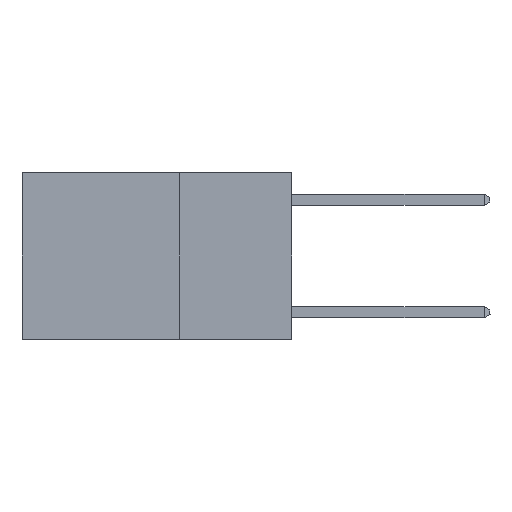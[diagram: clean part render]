
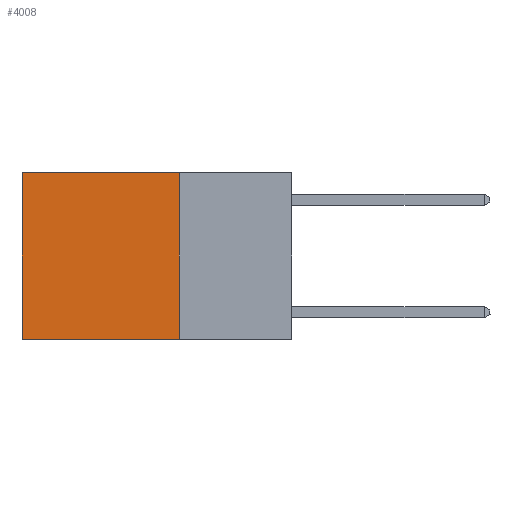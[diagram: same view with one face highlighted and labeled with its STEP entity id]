
A CAD part, left-side view. The second image highlights one B-rep face of the part: STEP entity #4008.
In plain terms, the highlighted planar face has unit normal (-1, 0, 0).
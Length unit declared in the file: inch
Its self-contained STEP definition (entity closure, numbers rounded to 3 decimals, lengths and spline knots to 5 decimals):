
#190 = VECTOR ( 'NONE', #16484, 39.37008 ) ;
#302 = CARTESIAN_POINT ( 'NONE',  ( 0.2625, 0.6, 0. ) ) ;
#377 = CARTESIAN_POINT ( 'NONE',  ( 0.2625, 0.6, -0.37 ) ) ;
#729 = EDGE_CURVE ( 'NONE', #3782, #8922, #2511, .T. ) ;
#951 = DIRECTION ( 'NONE',  ( 0., 0., -1. ) ) ;
#1135 = VECTOR ( 'NONE', #10407, 39.37008 ) ;
#2511 = LINE ( 'NONE', #17663, #1135 ) ;
#3301 = EDGE_CURVE ( 'NONE', #3782, #17445, #7290, .T. ) ;
#3782 = VERTEX_POINT ( 'NONE', #13985 ) ;
#4008 = ADVANCED_FACE ( 'NONE', ( #11550 ), #12716, .F. ) ;
#4341 = DIRECTION ( 'NONE',  ( 0., 1., 0. ) ) ;
#5199 = VERTEX_POINT ( 'NONE', #377 ) ;
#5431 = AXIS2_PLACEMENT_3D ( 'NONE', #18724, #9845, #951 ) ;
#5867 = CARTESIAN_POINT ( 'NONE',  ( 0.2625, 0.25, 0. ) ) ;
#6741 = ORIENTED_EDGE ( 'NONE', *, *, #8431, .F. ) ;
#6955 = ORIENTED_EDGE ( 'NONE', *, *, #729, .F. ) ;
#7290 = LINE ( 'NONE', #5867, #190 ) ;
#8431 = EDGE_CURVE ( 'NONE', #8922, #5199, #19445, .T. ) ;
#8922 = VERTEX_POINT ( 'NONE', #10956 ) ;
#9041 = ORIENTED_EDGE ( 'NONE', *, *, #3301, .T. ) ;
#9845 = DIRECTION ( 'NONE',  ( 1., 0., 0. ) ) ;
#10407 = DIRECTION ( 'NONE',  ( 0., 0., -1. ) ) ;
#10956 = CARTESIAN_POINT ( 'NONE',  ( 0.2625, 0.25, -0.37 ) ) ;
#11171 = DIRECTION ( 'NONE',  ( 0., 0., -1. ) ) ;
#11550 = FACE_OUTER_BOUND ( 'NONE', #15738, .T. ) ;
#11964 = CARTESIAN_POINT ( 'NONE',  ( 0.2625, 0.25, -0.37 ) ) ;
#12335 = EDGE_CURVE ( 'NONE', #17445, #5199, #12632, .T. ) ;
#12632 = LINE ( 'NONE', #18534, #18216 ) ;
#12716 = PLANE ( 'NONE',  #5431 ) ;
#12751 = ORIENTED_EDGE ( 'NONE', *, *, #12335, .T. ) ;
#13241 = VECTOR ( 'NONE', #4341, 39.37008 ) ;
#13985 = CARTESIAN_POINT ( 'NONE',  ( 0.2625, 0.25, 0. ) ) ;
#15738 = EDGE_LOOP ( 'NONE', ( #12751, #6741, #6955, #9041 ) ) ;
#16484 = DIRECTION ( 'NONE',  ( 0., 1., 0. ) ) ;
#17445 = VERTEX_POINT ( 'NONE', #302 ) ;
#17663 = CARTESIAN_POINT ( 'NONE',  ( 0.2625, 0.25, 0. ) ) ;
#18216 = VECTOR ( 'NONE', #11171, 39.37008 ) ;
#18534 = CARTESIAN_POINT ( 'NONE',  ( 0.2625, 0.6, 0. ) ) ;
#18724 = CARTESIAN_POINT ( 'NONE',  ( 0.2625, 0.25, 0. ) ) ;
#19445 = LINE ( 'NONE', #11964, #13241 ) ;
